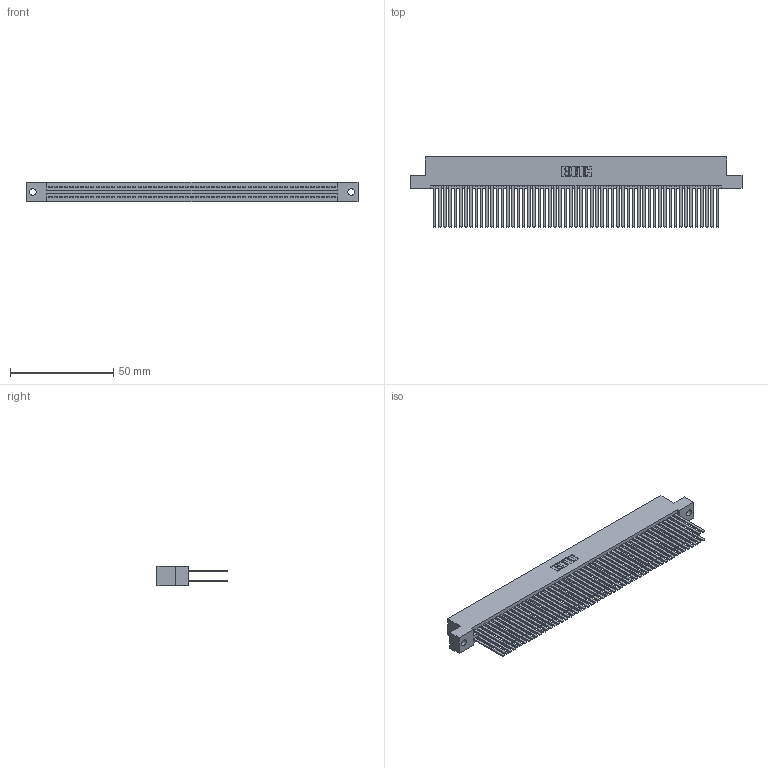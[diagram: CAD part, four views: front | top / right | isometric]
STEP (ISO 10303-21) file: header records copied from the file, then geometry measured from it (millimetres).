
FILE_DESCRIPTION (( 'STEP AP203' ), '1' );
FILE_NAME ('395-110-544-202.STEP', '2019-10-27T11:19:10', ( '' ), ( '' ), 'SwSTEP 2.0', 'SolidWorks 2016', '' );
FILE_SCHEMA (( 'CONFIG_CONTROL_DESIGN' ));
Length unit declared in the file: inch
Products named in the file (3): 345 Part_Flush Mounting Lugs - 0.128 Dia; 345-292-001_345-293-144; 395-110-544-202
Assembly tree (111 placements, depth 2):
  395-110-544-202
    345 Part_Flush Mounting Lugs - 0.128 Dia
    345-292-001_345-293-144  x110
Bounding box: 160.91 x 33.96 x 9.4 mm (x, y, z)
Volume: 17256.8 mm3; surface area: 30007 mm2
Topology: 111 solids, 111 shells, 4966 faces, 14751 edges, 9686 vertices
Faces by surface type: plane 3270, cylinder 1696
Entity records: 41223 total; most frequent: CARTESIAN_POINT 6896, ORIENTED_EDGE 6830, DIRECTION 6063, EDGE_CURVE 3415, VECTOR 3067, LINE 3067, VERTEX_POINT 2274, AXIS2_PLACEMENT_3D 1498
